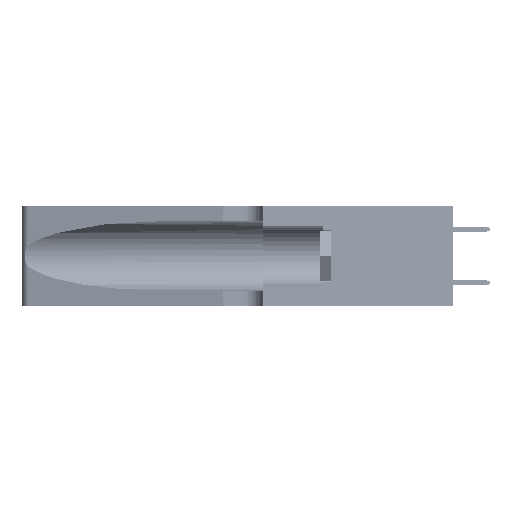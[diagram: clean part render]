
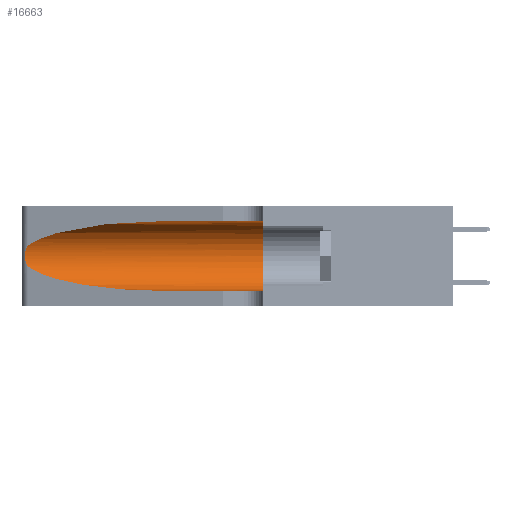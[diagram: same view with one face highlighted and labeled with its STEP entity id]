
A CAD part, left-side view. The second image highlights one B-rep face of the part: STEP entity #16663.
In plain terms, the highlighted cylindrical face has radius 3.308 mm (diameter 6.617 mm), a partial arc.
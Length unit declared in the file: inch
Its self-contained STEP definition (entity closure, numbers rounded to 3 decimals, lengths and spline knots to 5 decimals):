
#1635 = CARTESIAN_POINT ( 'NONE',  ( 0.25854, 1.2359, 0.20912 ) ) ;
#2446 = VECTOR ( 'NONE', #40541, 39.37008 ) ;
#2981 = CARTESIAN_POINT ( 'NONE',  ( 0.1305, 1.61858, 0.185 ) ) ;
#3300 = EDGE_CURVE ( 'NONE', #32444, #14505, #45430, .T. ) ;
#3440 = CARTESIAN_POINT ( 'NONE',  ( 0.2373, 1.15595, 0.08982 ) ) ;
#3928 = VERTEX_POINT ( 'NONE', #13698 ) ;
#4509 = CARTESIAN_POINT ( 'NONE',  ( 0.1305, 0.72297, 0.05475 ) ) ;
#4714 = EDGE_CURVE ( 'NONE', #5824, #7023, #33986, .T. ) ;
#5491 = CARTESIAN_POINT ( 'NONE',  ( 0.25856, 1.23593, 0.16098 ) ) ;
#5756 = CARTESIAN_POINT ( 'NONE',  ( 0.25555, 1.22994, 0.2215 ) ) ;
#5824 = VERTEX_POINT ( 'NONE', #12972 ) ;
#5871 = EDGE_LOOP ( 'NONE', ( #30731, #30251, #49062, #43405, #28280, #26517 ) ) ;
#6586 = DIRECTION ( 'NONE',  ( 0., 0., -1. ) ) ;
#7023 = VERTEX_POINT ( 'NONE', #13803 ) ;
#7474 = CARTESIAN_POINT ( 'NONE',  ( 0.1305, 0.35, 0.05475 ) ) ;
#8598 = CARTESIAN_POINT ( 'NONE',  ( 0.26017, 1.23833, 0.17102 ) ) ;
#8903 = CARTESIAN_POINT ( 'NONE',  ( 0.1305, 0.72297, 0.31525 ) ) ;
#10052 = CARTESIAN_POINT ( 'NONE',  ( 0.1305, 1.61858, 0.31525 ) ) ;
#12972 = CARTESIAN_POINT ( 'NONE',  ( 0.1305, 0.72297, 0.31525 ) ) ;
#13182 = CARTESIAN_POINT ( 'NONE',  ( 0.25639, 1.23186, 0.15144 ) ) ;
#13248 = CARTESIAN_POINT ( 'NONE',  ( 0.2373, 1.15595, 0.28018 ) ) ;
#13698 = CARTESIAN_POINT ( 'NONE',  ( 0.25487, 1.22718, 0.14631 ) ) ;
#13803 = CARTESIAN_POINT ( 'NONE',  ( 0.25487, 1.22718, 0.22369 ) ) ;
#14505 = VERTEX_POINT ( 'NONE', #7474 ) ;
#14767 = CYLINDRICAL_SURFACE ( 'NONE', #44987, 0.13025 ) ;
#15526 = DIRECTION ( 'NONE',  ( 0., -1., 0. ) ) ;
#16663 = ADVANCED_FACE ( 'NONE', ( #38586 ), #14767, .F. ) ;
#17555 = CARTESIAN_POINT ( 'NONE',  ( 0.25487, 1.22718, 0.14631 ) ) ;
#17984 = LINE ( 'NONE', #10052, #50008 ) ;
#19057 = CARTESIAN_POINT ( 'NONE',  ( 0.1305, 0.35, 0.31525 ) ) ;
#19109 = CARTESIAN_POINT ( 'NONE',  ( 0.1305, 0.72297, 0.05475 ) ) ;
#21789 = B_SPLINE_CURVE_WITH_KNOTS ( 'NONE', 3,
 ( #32347, #5756, #24820, #28450, #1635, #48348, #32842, #25076, #8598, #5491, #40361, #13182, #40626, #17555 ),
 .UNSPECIFIED., .F., .F.,
 ( 4, 2, 2, 2, 2, 2, 4 ),
 ( 0., 0.00027, 0.00053, 0.00107, 0.0016, 0.00187, 0.00214 ),
 .UNSPECIFIED. ) ;
#21887 = CARTESIAN_POINT ( 'NONE',  ( 0.1305, 1.61858, 0.05475 ) ) ;
#22486 = CARTESIAN_POINT ( 'NONE',  ( 0.18966, 0.96281, 0.05475 ) ) ;
#24820 = CARTESIAN_POINT ( 'NONE',  ( 0.25639, 1.23184, 0.21858 ) ) ;
#24856 = VERTEX_POINT ( 'NONE', #19057 ) ;
#24858 = EDGE_CURVE ( 'NONE', #24856, #14505, #42339, .T. ) ;
#25037 =( BOUNDED_CURVE ( )  B_SPLINE_CURVE ( 3, ( #26371, #3440, #22486, #19109 ),
 .UNSPECIFIED., .F., .T. ) 
 B_SPLINE_CURVE_WITH_KNOTS ( ( 4, 4 ),
 ( 3.44316, 4.71239 ),
 .UNSPECIFIED. ) 
 CURVE ( )  GEOMETRIC_REPRESENTATION_ITEM ( )  RATIONAL_B_SPLINE_CURVE ( ( 1., 0.87, 0.87, 1. ) ) 
 REPRESENTATION_ITEM ( '' )  );
#25076 = CARTESIAN_POINT ( 'NONE',  ( 0.26075, 1.23896, 0.178 ) ) ;
#26371 = CARTESIAN_POINT ( 'NONE',  ( 0.25487, 1.22718, 0.14631 ) ) ;
#26517 = ORIENTED_EDGE ( 'NONE', *, *, #38830, .F. ) ;
#28280 = ORIENTED_EDGE ( 'NONE', *, *, #24858, .F. ) ;
#28450 = CARTESIAN_POINT ( 'NONE',  ( 0.25787, 1.23484, 0.2124 ) ) ;
#29272 = CARTESIAN_POINT ( 'NONE',  ( 0.18966, 0.96281, 0.31525 ) ) ;
#30251 = ORIENTED_EDGE ( 'NONE', *, *, #44353, .T. ) ;
#30731 = ORIENTED_EDGE ( 'NONE', *, *, #4714, .T. ) ;
#32347 = CARTESIAN_POINT ( 'NONE',  ( 0.25487, 1.22718, 0.22369 ) ) ;
#32444 = VERTEX_POINT ( 'NONE', #4509 ) ;
#32842 = CARTESIAN_POINT ( 'NONE',  ( 0.26075, 1.23896, 0.19203 ) ) ;
#33780 = DIRECTION ( 'NONE',  ( 0., -1., 0. ) ) ;
#33986 =( BOUNDED_CURVE ( )  B_SPLINE_CURVE ( 3, ( #8903, #29272, #13248, #44804 ),
 .UNSPECIFIED., .F., .T. ) 
 B_SPLINE_CURVE_WITH_KNOTS ( ( 4, 4 ),
 ( 1.5708, 2.84003 ),
 .UNSPECIFIED. ) 
 CURVE ( )  GEOMETRIC_REPRESENTATION_ITEM ( )  RATIONAL_B_SPLINE_CURVE ( ( 1., 0.87, 0.87, 1. ) ) 
 REPRESENTATION_ITEM ( '' )  );
#35741 = AXIS2_PLACEMENT_3D ( 'NONE', #46737, #50585, #42863 ) ;
#38586 = FACE_OUTER_BOUND ( 'NONE', #5871, .T. ) ;
#38830 = EDGE_CURVE ( 'NONE', #5824, #24856, #17984, .T. ) ;
#40361 = CARTESIAN_POINT ( 'NONE',  ( 0.25789, 1.23486, 0.15765 ) ) ;
#40541 = DIRECTION ( 'NONE',  ( 0., -1., 0. ) ) ;
#40626 = CARTESIAN_POINT ( 'NONE',  ( 0.25555, 1.22993, 0.14849 ) ) ;
#42339 = CIRCLE ( 'NONE', #35741, 0.13025 ) ;
#42863 = DIRECTION ( 'NONE',  ( 0., 0., 1. ) ) ;
#43405 = ORIENTED_EDGE ( 'NONE', *, *, #3300, .T. ) ;
#44353 = EDGE_CURVE ( 'NONE', #7023, #3928, #21789, .T. ) ;
#44804 = CARTESIAN_POINT ( 'NONE',  ( 0.25487, 1.22718, 0.22369 ) ) ;
#44987 = AXIS2_PLACEMENT_3D ( 'NONE', #2981, #15526, #6586 ) ;
#45430 = LINE ( 'NONE', #21887, #2446 ) ;
#46737 = CARTESIAN_POINT ( 'NONE',  ( 0.1305, 0.35, 0.185 ) ) ;
#48348 = CARTESIAN_POINT ( 'NONE',  ( 0.26018, 1.23835, 0.19895 ) ) ;
#49062 = ORIENTED_EDGE ( 'NONE', *, *, #50311, .T. ) ;
#50008 = VECTOR ( 'NONE', #33780, 39.37008 ) ;
#50311 = EDGE_CURVE ( 'NONE', #3928, #32444, #25037, .T. ) ;
#50585 = DIRECTION ( 'NONE',  ( 0., 1., 0. ) ) ;
